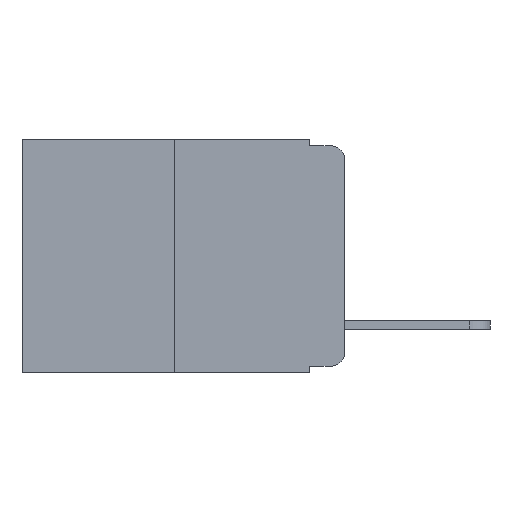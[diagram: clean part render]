
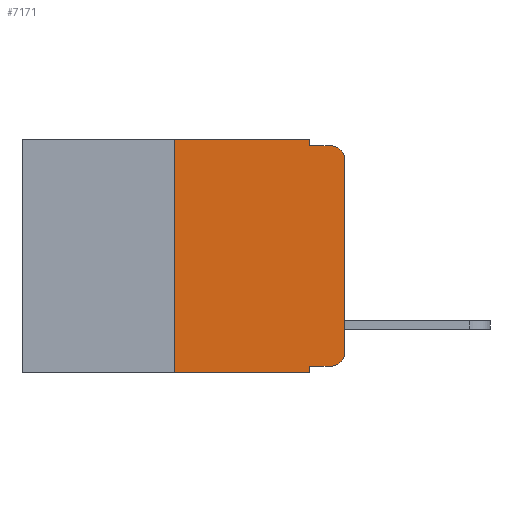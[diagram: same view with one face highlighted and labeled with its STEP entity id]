
A CAD part, left-side view. The second image highlights one B-rep face of the part: STEP entity #7171.
In plain terms, the highlighted planar face has unit normal (-1, 0, 0).
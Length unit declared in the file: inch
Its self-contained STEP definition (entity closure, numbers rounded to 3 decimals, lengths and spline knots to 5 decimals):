
#63 = ORIENTED_EDGE ( 'NONE', *, *, #18412, .F. ) ;
#229 = CARTESIAN_POINT ( 'NONE',  ( 0., 0., -0.313 ) ) ;
#348 = ORIENTED_EDGE ( 'NONE', *, *, #11782, .F. ) ;
#493 = CARTESIAN_POINT ( 'NONE',  ( 0., 0.051, -0.333 ) ) ;
#668 = CARTESIAN_POINT ( 'NONE',  ( 0., 0.02, -0.313 ) ) ;
#720 = VERTEX_POINT ( 'NONE', #9526 ) ;
#1246 = VECTOR ( 'NONE', #14022, 39.37008 ) ;
#1289 = EDGE_CURVE ( 'NONE', #5462, #4466, #5737, .T. ) ;
#2177 = DIRECTION ( 'NONE',  ( 0., -1., 0. ) ) ;
#2394 = CARTESIAN_POINT ( 'NONE',  ( 0., 0.051, 0. ) ) ;
#2400 = CARTESIAN_POINT ( 'NONE',  ( 0., 0.25, -0.343 ) ) ;
#2460 = DIRECTION ( 'NONE',  ( 0., 0., -1. ) ) ;
#2487 = CARTESIAN_POINT ( 'NONE',  ( 0., 0.051, 0. ) ) ;
#2976 = CARTESIAN_POINT ( 'NONE',  ( 0., 0.051, -0.343 ) ) ;
#3449 = DIRECTION ( 'NONE',  ( -1., 0., 0. ) ) ;
#3514 = DIRECTION ( 'NONE',  ( 0., 0., -1. ) ) ;
#3887 = FACE_OUTER_BOUND ( 'NONE', #19785, .T. ) ;
#4024 = CARTESIAN_POINT ( 'NONE',  ( 0., 0.473, 0. ) ) ;
#4185 = VECTOR ( 'NONE', #2177, 39.37008 ) ;
#4466 = VERTEX_POINT ( 'NONE', #14944 ) ;
#4686 = VERTEX_POINT ( 'NONE', #229 ) ;
#5002 = VERTEX_POINT ( 'NONE', #9505 ) ;
#5040 = VECTOR ( 'NONE', #14080, 39.37008 ) ;
#5462 = VERTEX_POINT ( 'NONE', #493 ) ;
#5512 = AXIS2_PLACEMENT_3D ( 'NONE', #14991, #3449, #3514 ) ;
#5614 = EDGE_CURVE ( 'NONE', #4686, #9665, #6088, .T. ) ;
#5708 = DIRECTION ( 'NONE',  ( -1., 0., 0. ) ) ;
#5737 = LINE ( 'NONE', #18731, #4185 ) ;
#5955 = ORIENTED_EDGE ( 'NONE', *, *, #13133, .F. ) ;
#6088 = LINE ( 'NONE', #14029, #18508 ) ;
#7091 = DIRECTION ( 'NONE',  ( 0., -1., 0. ) ) ;
#7171 = ADVANCED_FACE ( 'NONE', ( #3887 ), #16870, .F. ) ;
#7186 = LINE ( 'NONE', #2487, #1246 ) ;
#7592 = AXIS2_PLACEMENT_3D ( 'NONE', #4024, #9131, #15560 ) ;
#7756 = VERTEX_POINT ( 'NONE', #15517 ) ;
#7791 = EDGE_CURVE ( 'NONE', #4466, #4686, #9777, .T. ) ;
#8145 = EDGE_CURVE ( 'NONE', #12400, #720, #8237, .T. ) ;
#8237 = LINE ( 'NONE', #20451, #16491 ) ;
#9131 = DIRECTION ( 'NONE',  ( 1., 0., 0. ) ) ;
#9402 = CARTESIAN_POINT ( 'NONE',  ( 0., 0., -0.03 ) ) ;
#9505 = CARTESIAN_POINT ( 'NONE',  ( 0., 0.051, 0. ) ) ;
#9526 = CARTESIAN_POINT ( 'NONE',  ( 0., 0.02, -0.01 ) ) ;
#9665 = VERTEX_POINT ( 'NONE', #9402 ) ;
#9777 = CIRCLE ( 'NONE', #18948, 0.02 ) ;
#9795 = ORIENTED_EDGE ( 'NONE', *, *, #5614, .T. ) ;
#10575 = DIRECTION ( 'NONE',  ( 0., 0., 1. ) ) ;
#10742 = LINE ( 'NONE', #2394, #12825 ) ;
#11324 = ORIENTED_EDGE ( 'NONE', *, *, #8145, .F. ) ;
#11432 = ORIENTED_EDGE ( 'NONE', *, *, #7791, .T. ) ;
#11507 = LINE ( 'NONE', #16236, #19012 ) ;
#11782 = EDGE_CURVE ( 'NONE', #5462, #17122, #10742, .T. ) ;
#12400 = VERTEX_POINT ( 'NONE', #18707 ) ;
#12437 = CARTESIAN_POINT ( 'NONE',  ( 0., 0.473, -0.343 ) ) ;
#12825 = VECTOR ( 'NONE', #18732, 39.37008 ) ;
#13109 = VECTOR ( 'NONE', #16640, 39.37008 ) ;
#13133 = EDGE_CURVE ( 'NONE', #5002, #12400, #7186, .T. ) ;
#14022 = DIRECTION ( 'NONE',  ( 0., 0., -1. ) ) ;
#14029 = CARTESIAN_POINT ( 'NONE',  ( 0., 0., 0. ) ) ;
#14080 = DIRECTION ( 'NONE',  ( 0., -1., 0. ) ) ;
#14908 = CARTESIAN_POINT ( 'NONE',  ( 0., 0.25, 0. ) ) ;
#14944 = CARTESIAN_POINT ( 'NONE',  ( 0., 0.02, -0.333 ) ) ;
#14991 = CARTESIAN_POINT ( 'NONE',  ( 0., 0.02, -0.03 ) ) ;
#15453 = EDGE_CURVE ( 'NONE', #17009, #7756, #16204, .T. ) ;
#15517 = CARTESIAN_POINT ( 'NONE',  ( 0., 0.25, 0. ) ) ;
#15560 = DIRECTION ( 'NONE',  ( 0., 0., -1. ) ) ;
#16005 = EDGE_CURVE ( 'NONE', #9665, #720, #20340, .T. ) ;
#16041 = ORIENTED_EDGE ( 'NONE', *, *, #1289, .T. ) ;
#16204 = LINE ( 'NONE', #14908, #13109 ) ;
#16236 = CARTESIAN_POINT ( 'NONE',  ( 0., 0.473, 0. ) ) ;
#16396 = ORIENTED_EDGE ( 'NONE', *, *, #15453, .F. ) ;
#16491 = VECTOR ( 'NONE', #7091, 39.37008 ) ;
#16589 = ORIENTED_EDGE ( 'NONE', *, *, #16005, .T. ) ;
#16640 = DIRECTION ( 'NONE',  ( 0., 0., 1. ) ) ;
#16704 = ORIENTED_EDGE ( 'NONE', *, *, #17010, .T. ) ;
#16870 = PLANE ( 'NONE',  #7592 ) ;
#17009 = VERTEX_POINT ( 'NONE', #2400 ) ;
#17010 = EDGE_CURVE ( 'NONE', #17009, #17122, #21046, .T. ) ;
#17122 = VERTEX_POINT ( 'NONE', #2976 ) ;
#17913 = DIRECTION ( 'NONE',  ( 0., -1., 0. ) ) ;
#18412 = EDGE_CURVE ( 'NONE', #7756, #5002, #11507, .T. ) ;
#18508 = VECTOR ( 'NONE', #10575, 39.37008 ) ;
#18707 = CARTESIAN_POINT ( 'NONE',  ( 0., 0.051, -0.01 ) ) ;
#18731 = CARTESIAN_POINT ( 'NONE',  ( 0., 0.051, -0.333 ) ) ;
#18732 = DIRECTION ( 'NONE',  ( 0., 0., -1. ) ) ;
#18948 = AXIS2_PLACEMENT_3D ( 'NONE', #668, #5708, #2460 ) ;
#19012 = VECTOR ( 'NONE', #17913, 39.37008 ) ;
#19785 = EDGE_LOOP ( 'NONE', ( #9795, #16589, #11324, #5955, #63, #16396, #16704, #348, #16041, #11432 ) ) ;
#20340 = CIRCLE ( 'NONE', #5512, 0.02 ) ;
#20451 = CARTESIAN_POINT ( 'NONE',  ( 0., 0.051, -0.01 ) ) ;
#21046 = LINE ( 'NONE', #12437, #5040 ) ;
